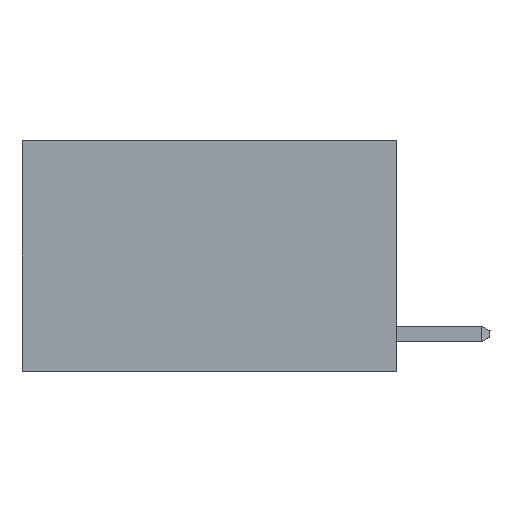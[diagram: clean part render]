
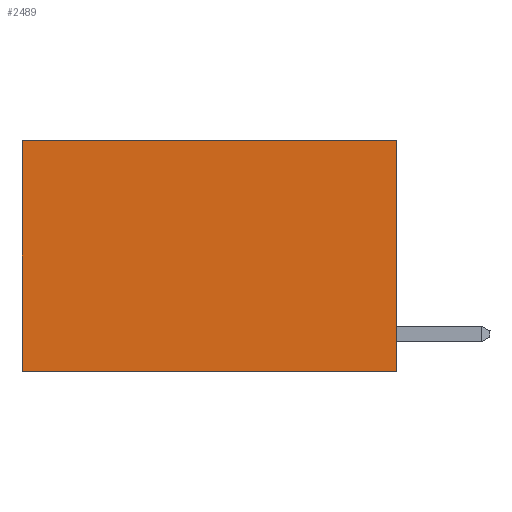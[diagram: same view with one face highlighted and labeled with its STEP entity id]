
A CAD part, left-side view. The second image highlights one B-rep face of the part: STEP entity #2489.
In plain terms, the highlighted planar face has unit normal (-1, 0, 0).
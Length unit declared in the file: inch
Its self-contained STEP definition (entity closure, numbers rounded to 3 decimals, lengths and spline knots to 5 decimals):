
#99 = LINE ( 'NONE', #20369, #6909 ) ;
#186 = VECTOR ( 'NONE', #8538, 39.37008 ) ;
#208 = VECTOR ( 'NONE', #4826, 39.37008 ) ;
#312 = CARTESIAN_POINT ( 'NONE',  ( 0.2625, 0.6, 0. ) ) ;
#434 = AXIS2_PLACEMENT_3D ( 'NONE', #17732, #14501, #16237 ) ;
#548 = DIRECTION ( 'NONE',  ( 0., 1., 0. ) ) ;
#1763 = ORIENTED_EDGE ( 'NONE', *, *, #5353, .T. ) ;
#2114 = EDGE_LOOP ( 'NONE', ( #1763, #18996, #9726, #15756 ) ) ;
#2489 = ADVANCED_FACE ( 'NONE', ( #14948 ), #19304, .F. ) ;
#2711 = VERTEX_POINT ( 'NONE', #9936 ) ;
#3557 = EDGE_CURVE ( 'NONE', #6678, #11299, #99, .T. ) ;
#4826 = DIRECTION ( 'NONE',  ( 0., 0., -1. ) ) ;
#5353 = EDGE_CURVE ( 'NONE', #11299, #12211, #5783, .T. ) ;
#5783 = LINE ( 'NONE', #9605, #14084 ) ;
#6494 = CARTESIAN_POINT ( 'NONE',  ( 0.2625, 0., 0. ) ) ;
#6678 = VERTEX_POINT ( 'NONE', #18420 ) ;
#6909 = VECTOR ( 'NONE', #548, 39.37008 ) ;
#8538 = DIRECTION ( 'NONE',  ( 0., 1., 0. ) ) ;
#9512 = CARTESIAN_POINT ( 'NONE',  ( 0.2625, 0.6, -0.37 ) ) ;
#9605 = CARTESIAN_POINT ( 'NONE',  ( 0.2625, 0.6, 0. ) ) ;
#9726 = ORIENTED_EDGE ( 'NONE', *, *, #18364, .F. ) ;
#9821 = LINE ( 'NONE', #19909, #186 ) ;
#9936 = CARTESIAN_POINT ( 'NONE',  ( 0.2625, 0., -0.37 ) ) ;
#11299 = VERTEX_POINT ( 'NONE', #312 ) ;
#12211 = VERTEX_POINT ( 'NONE', #9512 ) ;
#14084 = VECTOR ( 'NONE', #21140, 39.37008 ) ;
#14186 = EDGE_CURVE ( 'NONE', #2711, #12211, #9821, .T. ) ;
#14501 = DIRECTION ( 'NONE',  ( 1., 0., 0. ) ) ;
#14948 = FACE_OUTER_BOUND ( 'NONE', #2114, .T. ) ;
#15756 = ORIENTED_EDGE ( 'NONE', *, *, #3557, .T. ) ;
#16237 = DIRECTION ( 'NONE',  ( 0., 0., -1. ) ) ;
#17732 = CARTESIAN_POINT ( 'NONE',  ( 0.2625, 0., 0. ) ) ;
#18364 = EDGE_CURVE ( 'NONE', #6678, #2711, #20684, .T. ) ;
#18420 = CARTESIAN_POINT ( 'NONE',  ( 0.2625, 0., 0. ) ) ;
#18996 = ORIENTED_EDGE ( 'NONE', *, *, #14186, .F. ) ;
#19304 = PLANE ( 'NONE',  #434 ) ;
#19909 = CARTESIAN_POINT ( 'NONE',  ( 0.2625, 0., -0.37 ) ) ;
#20369 = CARTESIAN_POINT ( 'NONE',  ( 0.2625, 0., 0. ) ) ;
#20684 = LINE ( 'NONE', #6494, #208 ) ;
#21140 = DIRECTION ( 'NONE',  ( 0., 0., -1. ) ) ;
